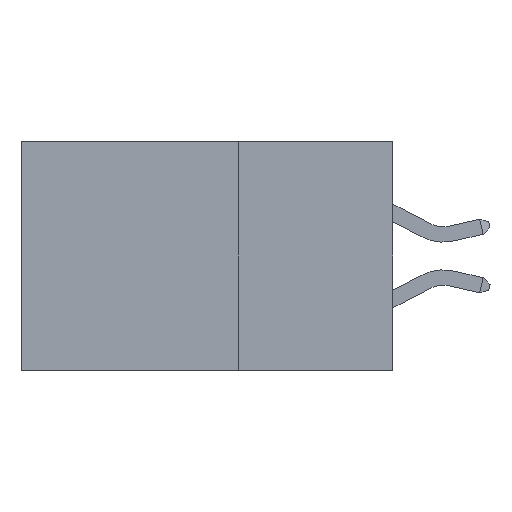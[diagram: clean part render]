
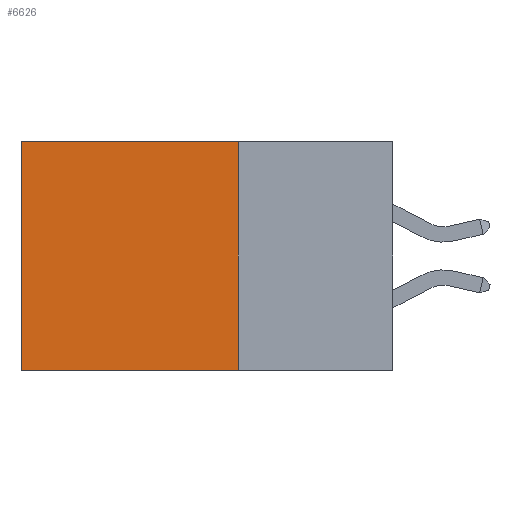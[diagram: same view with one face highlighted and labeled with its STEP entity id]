
A CAD part, left-side view. The second image highlights one B-rep face of the part: STEP entity #6626.
In plain terms, the highlighted planar face has unit normal (-1, 0, 0).
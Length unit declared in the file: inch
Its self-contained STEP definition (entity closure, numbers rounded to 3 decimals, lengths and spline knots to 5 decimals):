
#637 = DIRECTION ( 'NONE',  ( 0., 1., 0. ) ) ;
#710 = VECTOR ( 'NONE', #1833, 39.37008 ) ;
#731 = AXIS2_PLACEMENT_3D ( 'NONE', #12055, #5755, #13110 ) ;
#919 = LINE ( 'NONE', #13488, #13363 ) ;
#1059 = LINE ( 'NONE', #4404, #710 ) ;
#1594 = DIRECTION ( 'NONE',  ( 0., 0., -1. ) ) ;
#1833 = DIRECTION ( 'NONE',  ( 0., 0., -1. ) ) ;
#2625 = PLANE ( 'NONE',  #731 ) ;
#2652 = CARTESIAN_POINT ( 'NONE',  ( 0.2875, 0.25, -0.37 ) ) ;
#2654 = CARTESIAN_POINT ( 'NONE',  ( 0.2875, 0.25, 0. ) ) ;
#2856 = EDGE_CURVE ( 'NONE', #6840, #11880, #13231, .T. ) ;
#3667 = EDGE_CURVE ( 'NONE', #11880, #3919, #8094, .T. ) ;
#3919 = VERTEX_POINT ( 'NONE', #8337 ) ;
#4404 = CARTESIAN_POINT ( 'NONE',  ( 0.2875, 0.6, 0. ) ) ;
#5247 = ORIENTED_EDGE ( 'NONE', *, *, #2856, .F. ) ;
#5480 = EDGE_LOOP ( 'NONE', ( #6908, #8107, #5247, #7167 ) ) ;
#5755 = DIRECTION ( 'NONE',  ( 1., 0., 0. ) ) ;
#6144 = VECTOR ( 'NONE', #1594, 39.37008 ) ;
#6432 = CARTESIAN_POINT ( 'NONE',  ( 0.2875, 0.25, -0.37 ) ) ;
#6626 = ADVANCED_FACE ( 'NONE', ( #11232 ), #2625, .F. ) ;
#6757 = EDGE_CURVE ( 'NONE', #6840, #12336, #919, .T. ) ;
#6840 = VERTEX_POINT ( 'NONE', #7454 ) ;
#6908 = ORIENTED_EDGE ( 'NONE', *, *, #7890, .T. ) ;
#7167 = ORIENTED_EDGE ( 'NONE', *, *, #6757, .T. ) ;
#7454 = CARTESIAN_POINT ( 'NONE',  ( 0.2875, 0.25, 0. ) ) ;
#7890 = EDGE_CURVE ( 'NONE', #12336, #3919, #1059, .T. ) ;
#8094 = LINE ( 'NONE', #2652, #11590 ) ;
#8107 = ORIENTED_EDGE ( 'NONE', *, *, #3667, .F. ) ;
#8337 = CARTESIAN_POINT ( 'NONE',  ( 0.2875, 0.6, -0.37 ) ) ;
#8375 = DIRECTION ( 'NONE',  ( 0., 1., 0. ) ) ;
#10477 = CARTESIAN_POINT ( 'NONE',  ( 0.2875, 0.6, 0. ) ) ;
#11232 = FACE_OUTER_BOUND ( 'NONE', #5480, .T. ) ;
#11590 = VECTOR ( 'NONE', #637, 39.37008 ) ;
#11880 = VERTEX_POINT ( 'NONE', #6432 ) ;
#12055 = CARTESIAN_POINT ( 'NONE',  ( 0.2875, 0.25, 0. ) ) ;
#12336 = VERTEX_POINT ( 'NONE', #10477 ) ;
#13110 = DIRECTION ( 'NONE',  ( 0., 0., -1. ) ) ;
#13231 = LINE ( 'NONE', #2654, #6144 ) ;
#13363 = VECTOR ( 'NONE', #8375, 39.37008 ) ;
#13488 = CARTESIAN_POINT ( 'NONE',  ( 0.2875, 0.25, 0. ) ) ;
